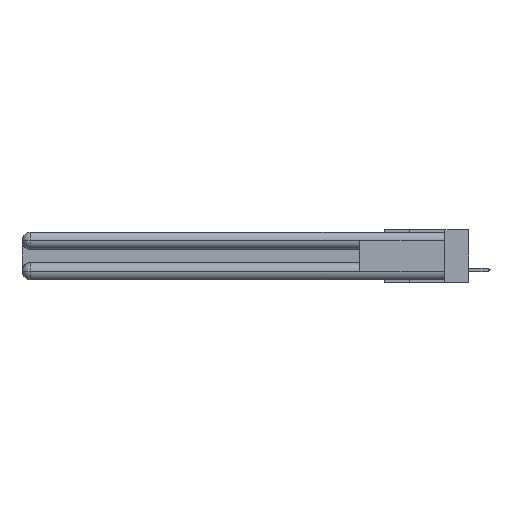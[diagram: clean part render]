
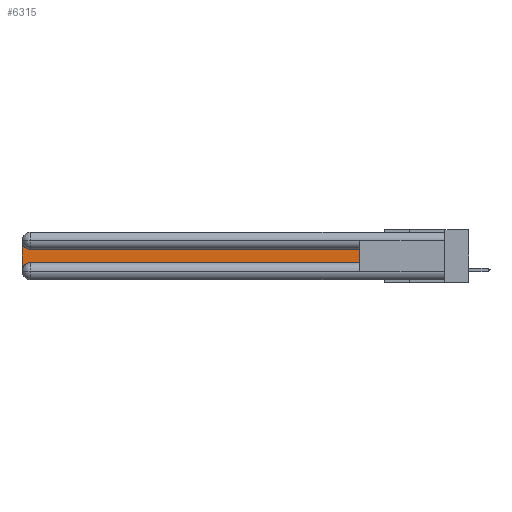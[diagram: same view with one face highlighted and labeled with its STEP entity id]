
A CAD part, left-side view. The second image highlights one B-rep face of the part: STEP entity #6315.
In plain terms, the highlighted planar face has unit normal (-1, 0, 0).
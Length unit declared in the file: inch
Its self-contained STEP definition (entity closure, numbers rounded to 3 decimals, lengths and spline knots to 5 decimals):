
#1188 = EDGE_CURVE ( 'NONE', #26940, #2734, #29883, .T. ) ;
#1592 = CARTESIAN_POINT ( 'NONE',  ( 0.075, 3., -0.2775 ) ) ;
#2734 = VERTEX_POINT ( 'NONE', #9910 ) ;
#3260 = CARTESIAN_POINT ( 'NONE',  ( 0.075, 3., -0.2175 ) ) ;
#3590 = EDGE_CURVE ( 'NONE', #6228, #15507, #27007, .T. ) ;
#3716 = VECTOR ( 'NONE', #9498, 39.37008 ) ;
#4088 = EDGE_CURVE ( 'NONE', #27605, #6228, #10367, .T. ) ;
#4232 = CARTESIAN_POINT ( 'NONE',  ( 0.075, 0.6, -0.1225 ) ) ;
#5998 = ORIENTED_EDGE ( 'NONE', *, *, #19977, .T. ) ;
#6009 = CARTESIAN_POINT ( 'NONE',  ( 0.075, 2.94, -0.2775 ) ) ;
#6228 = VERTEX_POINT ( 'NONE', #20828 ) ;
#6315 = ADVANCED_FACE ( 'NONE', ( #27733 ), #15237, .F. ) ;
#6317 = DIRECTION ( 'NONE',  ( 1., 0., 0. ) ) ;
#6544 = CARTESIAN_POINT ( 'NONE',  ( 0.075, 3., -0.1225 ) ) ;
#9498 = DIRECTION ( 'NONE',  ( 0., 1., 0. ) ) ;
#9736 = CIRCLE ( 'NONE', #11807, 0.06 ) ;
#9910 = CARTESIAN_POINT ( 'NONE',  ( 0.075, 0.6, -0.2175 ) ) ;
#10367 = CIRCLE ( 'NONE', #12184, 0.06 ) ;
#10877 = DIRECTION ( 'NONE',  ( 0., 0., -1. ) ) ;
#11189 = ORIENTED_EDGE ( 'NONE', *, *, #24046, .T. ) ;
#11545 = DIRECTION ( 'NONE',  ( 1., 0., 0. ) ) ;
#11807 = AXIS2_PLACEMENT_3D ( 'NONE', #6009, #6317, #23632 ) ;
#11913 = CARTESIAN_POINT ( 'NONE',  ( 0.075, 0.6, -0.2175 ) ) ;
#12184 = AXIS2_PLACEMENT_3D ( 'NONE', #19851, #22346, #10877 ) ;
#12246 = LINE ( 'NONE', #12304, #23490 ) ;
#12304 = CARTESIAN_POINT ( 'NONE',  ( 0.075, 0.6, -0.2175 ) ) ;
#13470 = LINE ( 'NONE', #24102, #3716 ) ;
#15237 = PLANE ( 'NONE',  #30721 ) ;
#15507 = VERTEX_POINT ( 'NONE', #1592 ) ;
#15698 = ORIENTED_EDGE ( 'NONE', *, *, #1188, .T. ) ;
#16306 = VECTOR ( 'NONE', #21423, 39.37008 ) ;
#17737 = EDGE_CURVE ( 'NONE', #15507, #26940, #9736, .T. ) ;
#17865 = CARTESIAN_POINT ( 'NONE',  ( 0.075, 2.94, -0.1225 ) ) ;
#19394 = EDGE_LOOP ( 'NONE', ( #5998, #27265, #29817, #28153, #15698, #11189 ) ) ;
#19851 = CARTESIAN_POINT ( 'NONE',  ( 0.075, 2.94, -0.0625 ) ) ;
#19977 = EDGE_CURVE ( 'NONE', #21072, #27605, #13470, .T. ) ;
#20828 = CARTESIAN_POINT ( 'NONE',  ( 0.075, 3., -0.0625 ) ) ;
#21072 = VERTEX_POINT ( 'NONE', #4232 ) ;
#21423 = DIRECTION ( 'NONE',  ( 0., -1., 0. ) ) ;
#21468 = CARTESIAN_POINT ( 'NONE',  ( 0.075, 2.94, -0.2175 ) ) ;
#22346 = DIRECTION ( 'NONE',  ( 1., 0., 0. ) ) ;
#23490 = VECTOR ( 'NONE', #32144, 39.37008 ) ;
#23632 = DIRECTION ( 'NONE',  ( 0., 0., -1. ) ) ;
#24046 = EDGE_CURVE ( 'NONE', #2734, #21072, #12246, .T. ) ;
#24102 = CARTESIAN_POINT ( 'NONE',  ( 0.075, 0.6, -0.1225 ) ) ;
#26561 = DIRECTION ( 'NONE',  ( 0., 0., -1. ) ) ;
#26940 = VERTEX_POINT ( 'NONE', #21468 ) ;
#27007 = LINE ( 'NONE', #3260, #27822 ) ;
#27265 = ORIENTED_EDGE ( 'NONE', *, *, #4088, .T. ) ;
#27605 = VERTEX_POINT ( 'NONE', #17865 ) ;
#27733 = FACE_OUTER_BOUND ( 'NONE', #19394, .T. ) ;
#27822 = VECTOR ( 'NONE', #28315, 39.37008 ) ;
#28153 = ORIENTED_EDGE ( 'NONE', *, *, #17737, .T. ) ;
#28315 = DIRECTION ( 'NONE',  ( 0., 0., -1. ) ) ;
#29817 = ORIENTED_EDGE ( 'NONE', *, *, #3590, .T. ) ;
#29883 = LINE ( 'NONE', #11913, #16306 ) ;
#30721 = AXIS2_PLACEMENT_3D ( 'NONE', #6544, #11545, #26561 ) ;
#32144 = DIRECTION ( 'NONE',  ( 0., 0., 1. ) ) ;
